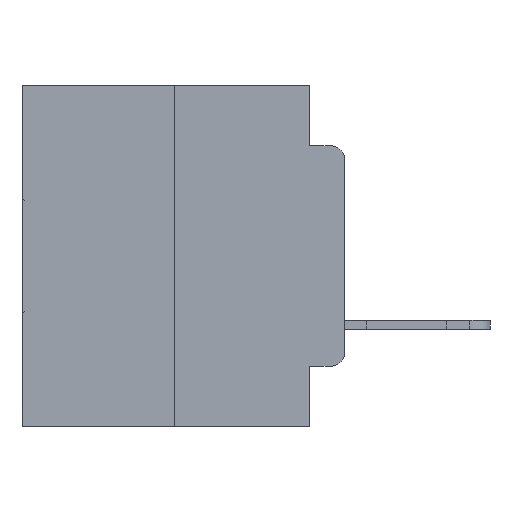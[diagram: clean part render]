
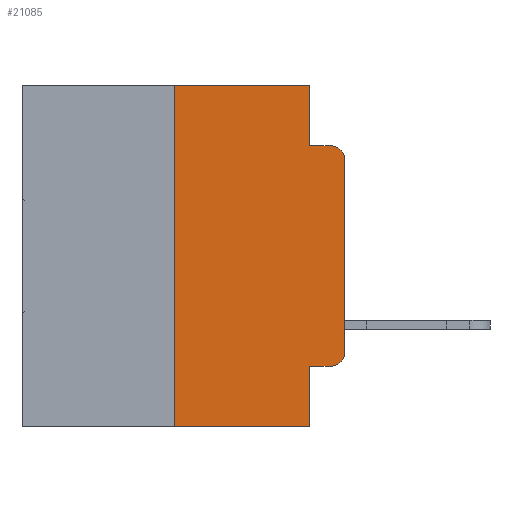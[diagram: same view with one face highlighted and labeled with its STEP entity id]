
A CAD part, left-side view. The second image highlights one B-rep face of the part: STEP entity #21085.
In plain terms, the highlighted planar face has unit normal (-1, 0, 0).
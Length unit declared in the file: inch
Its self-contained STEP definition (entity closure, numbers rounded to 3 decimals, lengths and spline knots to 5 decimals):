
#23 = DIRECTION ( 'NONE',  ( 0., 0., -1. ) ) ;
#50 = VECTOR ( 'NONE', #23, 39.37008 ) ;
#118 = ORIENTED_EDGE ( 'NONE', *, *, #11792, .F. ) ;
#462 = PLANE ( 'NONE',  #4852 ) ;
#706 = DIRECTION ( 'NONE',  ( 0., 0., -1. ) ) ;
#1171 = VERTEX_POINT ( 'NONE', #5957 ) ;
#1788 = EDGE_CURVE ( 'NONE', #27968, #5466, #7838, .T. ) ;
#2119 = DIRECTION ( 'NONE',  ( 0., -1., 0. ) ) ;
#2365 = VERTEX_POINT ( 'NONE', #19971 ) ;
#3557 = VERTEX_POINT ( 'NONE', #29083 ) ;
#4019 = FACE_OUTER_BOUND ( 'NONE', #14961, .T. ) ;
#4254 = ORIENTED_EDGE ( 'NONE', *, *, #28289, .T. ) ;
#4774 = CARTESIAN_POINT ( 'NONE',  ( 0., 0.051, -0.4115 ) ) ;
#4836 = EDGE_CURVE ( 'NONE', #3557, #26457, #13886, .T. ) ;
#4852 = AXIS2_PLACEMENT_3D ( 'NONE', #12354, #19261, #5333 ) ;
#4867 = CARTESIAN_POINT ( 'NONE',  ( 0., 0.051, 0. ) ) ;
#4950 = CARTESIAN_POINT ( 'NONE',  ( 0., 0.02, -0.1085 ) ) ;
#5333 = DIRECTION ( 'NONE',  ( 0., 0., -1. ) ) ;
#5466 = VERTEX_POINT ( 'NONE', #25806 ) ;
#5683 = EDGE_CURVE ( 'NONE', #3557, #2365, #27214, .T. ) ;
#5957 = CARTESIAN_POINT ( 'NONE',  ( 0., 0.02, -0.4115 ) ) ;
#6033 = CARTESIAN_POINT ( 'NONE',  ( 0., 0., -0.1085 ) ) ;
#6573 = CARTESIAN_POINT ( 'NONE',  ( 0., 0.473, 0. ) ) ;
#7235 = LINE ( 'NONE', #4867, #50 ) ;
#7350 = VECTOR ( 'NONE', #2119, 39.37008 ) ;
#7375 = ORIENTED_EDGE ( 'NONE', *, *, #5683, .F. ) ;
#7395 = DIRECTION ( 'NONE',  ( 0., 0., -1. ) ) ;
#7838 = LINE ( 'NONE', #29496, #8581 ) ;
#8118 = ORIENTED_EDGE ( 'NONE', *, *, #1788, .F. ) ;
#8447 = VECTOR ( 'NONE', #23179, 39.37008 ) ;
#8581 = VECTOR ( 'NONE', #13244, 39.37008 ) ;
#8903 = ORIENTED_EDGE ( 'NONE', *, *, #11418, .T. ) ;
#10175 = VERTEX_POINT ( 'NONE', #6033 ) ;
#10668 = ORIENTED_EDGE ( 'NONE', *, *, #4836, .T. ) ;
#11349 = CIRCLE ( 'NONE', #20270, 0.02 ) ;
#11418 = EDGE_CURVE ( 'NONE', #1171, #20048, #17565, .T. ) ;
#11792 = EDGE_CURVE ( 'NONE', #5466, #12151, #25604, .T. ) ;
#12151 = VERTEX_POINT ( 'NONE', #15276 ) ;
#12354 = CARTESIAN_POINT ( 'NONE',  ( 0., 0.473, 0. ) ) ;
#12715 = CARTESIAN_POINT ( 'NONE',  ( 0., 0., -0.3915 ) ) ;
#12871 = CARTESIAN_POINT ( 'NONE',  ( 0., 0., 0. ) ) ;
#13244 = DIRECTION ( 'NONE',  ( 0., 0., -1. ) ) ;
#13599 = VECTOR ( 'NONE', #15921, 39.37008 ) ;
#13647 = EDGE_CURVE ( 'NONE', #25032, #26457, #7235, .T. ) ;
#13886 = LINE ( 'NONE', #23505, #8447 ) ;
#14913 = DIRECTION ( 'NONE',  ( -1., 0., 0. ) ) ;
#14961 = EDGE_LOOP ( 'NONE', ( #4254, #14962, #118, #8118, #18582, #7375, #10668, #21022, #25565, #8903 ) ) ;
#14962 = ORIENTED_EDGE ( 'NONE', *, *, #19850, .T. ) ;
#15276 = CARTESIAN_POINT ( 'NONE',  ( 0., 0.02, -0.0885 ) ) ;
#15921 = DIRECTION ( 'NONE',  ( 0., -1., 0. ) ) ;
#16265 = CARTESIAN_POINT ( 'NONE',  ( 0., 0.051, -0.0885 ) ) ;
#17351 = VECTOR ( 'NONE', #18031, 39.37008 ) ;
#17565 = CIRCLE ( 'NONE', #17992, 0.02 ) ;
#17992 = AXIS2_PLACEMENT_3D ( 'NONE', #28286, #14913, #706 ) ;
#18031 = DIRECTION ( 'NONE',  ( 0., -1., 0. ) ) ;
#18582 = ORIENTED_EDGE ( 'NONE', *, *, #21987, .F. ) ;
#19261 = DIRECTION ( 'NONE',  ( 1., 0., 0. ) ) ;
#19850 = EDGE_CURVE ( 'NONE', #10175, #12151, #11349, .T. ) ;
#19971 = CARTESIAN_POINT ( 'NONE',  ( 0., 0.25, 0. ) ) ;
#20048 = VERTEX_POINT ( 'NONE', #12715 ) ;
#20270 = AXIS2_PLACEMENT_3D ( 'NONE', #4950, #21212, #7395 ) ;
#20419 = LINE ( 'NONE', #6573, #13599 ) ;
#20567 = DIRECTION ( 'NONE',  ( 0., 0., 1. ) ) ;
#20797 = CARTESIAN_POINT ( 'NONE',  ( 0., 0.051, 0. ) ) ;
#21022 = ORIENTED_EDGE ( 'NONE', *, *, #13647, .F. ) ;
#21085 = ADVANCED_FACE ( 'NONE', ( #4019 ), #462, .F. ) ;
#21212 = DIRECTION ( 'NONE',  ( -1., 0., 0. ) ) ;
#21260 = CARTESIAN_POINT ( 'NONE',  ( 0., 0.25, 0. ) ) ;
#21338 = VECTOR ( 'NONE', #20567, 39.37008 ) ;
#21978 = VECTOR ( 'NONE', #26424, 39.37008 ) ;
#21987 = EDGE_CURVE ( 'NONE', #2365, #27968, #20419, .T. ) ;
#23179 = DIRECTION ( 'NONE',  ( 0., -1., 0. ) ) ;
#23505 = CARTESIAN_POINT ( 'NONE',  ( 0., 0.473, -0.5 ) ) ;
#25032 = VERTEX_POINT ( 'NONE', #4774 ) ;
#25565 = ORIENTED_EDGE ( 'NONE', *, *, #26100, .T. ) ;
#25604 = LINE ( 'NONE', #16265, #7350 ) ;
#25806 = CARTESIAN_POINT ( 'NONE',  ( 0., 0.051, -0.0885 ) ) ;
#26100 = EDGE_CURVE ( 'NONE', #25032, #1171, #27761, .T. ) ;
#26154 = CARTESIAN_POINT ( 'NONE',  ( 0., 0.051, -0.5 ) ) ;
#26424 = DIRECTION ( 'NONE',  ( 0., 0., 1. ) ) ;
#26457 = VERTEX_POINT ( 'NONE', #26154 ) ;
#27214 = LINE ( 'NONE', #21260, #21338 ) ;
#27761 = LINE ( 'NONE', #29128, #17351 ) ;
#27775 = LINE ( 'NONE', #12871, #21978 ) ;
#27968 = VERTEX_POINT ( 'NONE', #20797 ) ;
#28286 = CARTESIAN_POINT ( 'NONE',  ( 0., 0.02, -0.3915 ) ) ;
#28289 = EDGE_CURVE ( 'NONE', #20048, #10175, #27775, .T. ) ;
#29083 = CARTESIAN_POINT ( 'NONE',  ( 0., 0.25, -0.5 ) ) ;
#29128 = CARTESIAN_POINT ( 'NONE',  ( 0., 0.051, -0.4115 ) ) ;
#29496 = CARTESIAN_POINT ( 'NONE',  ( 0., 0.051, 0. ) ) ;
